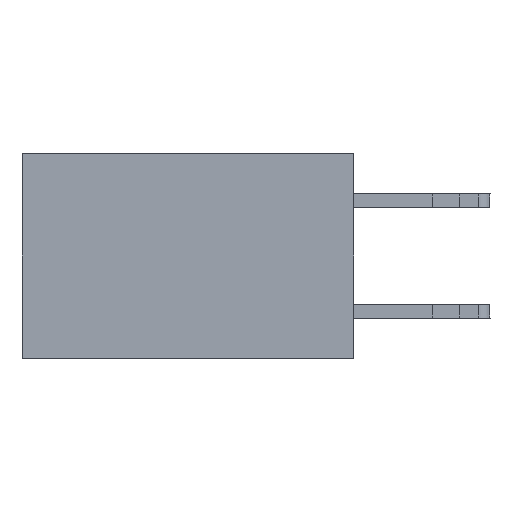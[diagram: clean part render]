
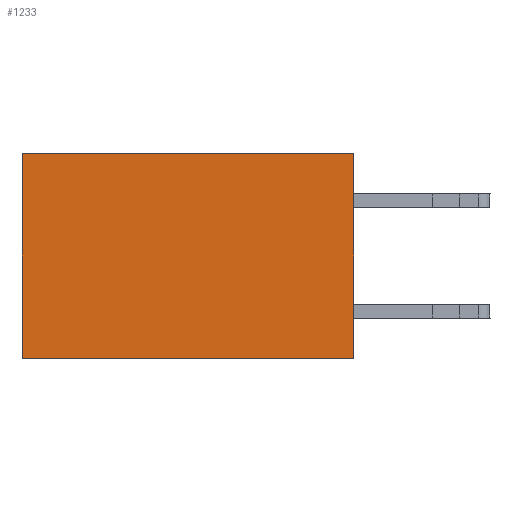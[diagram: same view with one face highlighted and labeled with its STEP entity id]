
A CAD part, left-side view. The second image highlights one B-rep face of the part: STEP entity #1233.
In plain terms, the highlighted planar face has unit normal (-1, 0, 0).
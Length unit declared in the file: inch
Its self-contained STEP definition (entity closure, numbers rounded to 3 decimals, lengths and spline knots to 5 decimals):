
#345 = CARTESIAN_POINT ( 'NONE',  ( 0.2875, 0.6, -0.37 ) ) ;
#1233 = ADVANCED_FACE ( 'NONE', ( #9638 ), #17697, .F. ) ;
#2062 = ORIENTED_EDGE ( 'NONE', *, *, #4512, .T. ) ;
#2532 = CARTESIAN_POINT ( 'NONE',  ( 0.2875, 0., 0. ) ) ;
#4183 = ORIENTED_EDGE ( 'NONE', *, *, #15433, .F. ) ;
#4512 = EDGE_CURVE ( 'NONE', #19088, #29727, #18030, .T. ) ;
#5329 = EDGE_CURVE ( 'NONE', #29727, #25596, #19461, .T. ) ;
#5459 = CARTESIAN_POINT ( 'NONE',  ( 0.2875, 0., 0. ) ) ;
#5744 = VECTOR ( 'NONE', #14617, 39.37008 ) ;
#5775 = CARTESIAN_POINT ( 'NONE',  ( 0.2875, 0., 0. ) ) ;
#6417 = ORIENTED_EDGE ( 'NONE', *, *, #7155, .F. ) ;
#6925 = CARTESIAN_POINT ( 'NONE',  ( 0.2875, 0., -0.37 ) ) ;
#7155 = EDGE_CURVE ( 'NONE', #27207, #25596, #21176, .T. ) ;
#7545 = DIRECTION ( 'NONE',  ( 0., 1., 0. ) ) ;
#9223 = VECTOR ( 'NONE', #7545, 39.37008 ) ;
#9251 = CARTESIAN_POINT ( 'NONE',  ( 0.2875, 0.6, 0. ) ) ;
#9638 = FACE_OUTER_BOUND ( 'NONE', #25142, .T. ) ;
#14054 = VECTOR ( 'NONE', #15946, 39.37008 ) ;
#14617 = DIRECTION ( 'NONE',  ( 0., 0., -1. ) ) ;
#15207 = CARTESIAN_POINT ( 'NONE',  ( 0.2875, 0., 0. ) ) ;
#15433 = EDGE_CURVE ( 'NONE', #19088, #27207, #18785, .T. ) ;
#15946 = DIRECTION ( 'NONE',  ( 0., 0., -1. ) ) ;
#17513 = DIRECTION ( 'NONE',  ( 0., 1., 0. ) ) ;
#17697 = PLANE ( 'NONE',  #29629 ) ;
#18030 = LINE ( 'NONE', #5775, #23090 ) ;
#18785 = LINE ( 'NONE', #5459, #5744 ) ;
#19088 = VERTEX_POINT ( 'NONE', #2532 ) ;
#19461 = LINE ( 'NONE', #9251, #14054 ) ;
#21176 = LINE ( 'NONE', #6925, #9223 ) ;
#23090 = VECTOR ( 'NONE', #17513, 39.37008 ) ;
#24195 = CARTESIAN_POINT ( 'NONE',  ( 0.2875, 0.6, 0. ) ) ;
#24883 = ORIENTED_EDGE ( 'NONE', *, *, #5329, .T. ) ;
#25142 = EDGE_LOOP ( 'NONE', ( #24883, #6417, #4183, #2062 ) ) ;
#25596 = VERTEX_POINT ( 'NONE', #345 ) ;
#26825 = DIRECTION ( 'NONE',  ( 1., 0., 0. ) ) ;
#27207 = VERTEX_POINT ( 'NONE', #29017 ) ;
#29017 = CARTESIAN_POINT ( 'NONE',  ( 0.2875, 0., -0.37 ) ) ;
#29216 = DIRECTION ( 'NONE',  ( 0., 0., -1. ) ) ;
#29629 = AXIS2_PLACEMENT_3D ( 'NONE', #15207, #26825, #29216 ) ;
#29727 = VERTEX_POINT ( 'NONE', #24195 ) ;
